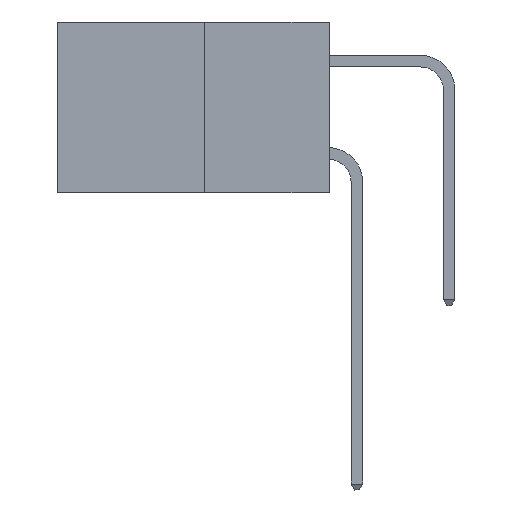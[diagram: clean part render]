
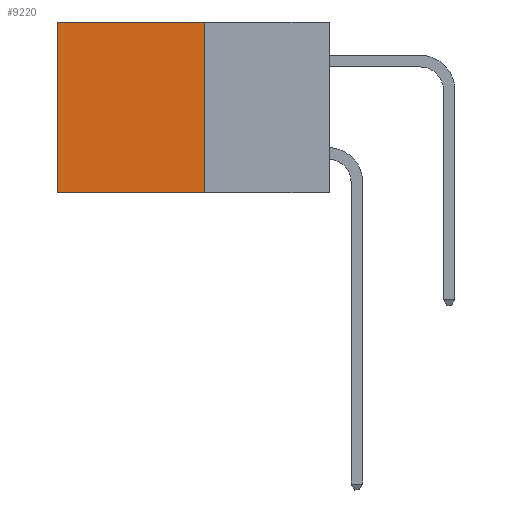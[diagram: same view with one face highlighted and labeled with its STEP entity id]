
A CAD part, left-side view. The second image highlights one B-rep face of the part: STEP entity #9220.
In plain terms, the highlighted planar face has unit normal (-1, 0, 0).
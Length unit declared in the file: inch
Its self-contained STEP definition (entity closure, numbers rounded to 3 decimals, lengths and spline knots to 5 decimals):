
#545 = VECTOR ( 'NONE', #9504, 39.37008 ) ;
#812 = LINE ( 'NONE', #10766, #545 ) ;
#907 = EDGE_CURVE ( 'NONE', #7436, #2865, #6226, .T. ) ;
#1232 = EDGE_CURVE ( 'NONE', #2865, #1827, #4604, .T. ) ;
#1278 = VECTOR ( 'NONE', #3513, 39.37008 ) ;
#1599 = CARTESIAN_POINT ( 'NONE',  ( 0.277, 0.27, 0. ) ) ;
#1723 = VERTEX_POINT ( 'NONE', #8814 ) ;
#1827 = VERTEX_POINT ( 'NONE', #4415 ) ;
#2842 = CARTESIAN_POINT ( 'NONE',  ( 0.277, 0.27, -0.37 ) ) ;
#2865 = VERTEX_POINT ( 'NONE', #7049 ) ;
#2949 = ORIENTED_EDGE ( 'NONE', *, *, #3234, .T. ) ;
#3029 = ORIENTED_EDGE ( 'NONE', *, *, #6302, .T. ) ;
#3068 = ORIENTED_EDGE ( 'NONE', *, *, #1232, .F. ) ;
#3146 = VECTOR ( 'NONE', #5377, 39.37008 ) ;
#3234 = EDGE_CURVE ( 'NONE', #7436, #1723, #812, .T. ) ;
#3513 = DIRECTION ( 'NONE',  ( 0., 0., -1. ) ) ;
#3969 = ORIENTED_EDGE ( 'NONE', *, *, #907, .F. ) ;
#4068 = FACE_OUTER_BOUND ( 'NONE', #8256, .T. ) ;
#4148 = CARTESIAN_POINT ( 'NONE',  ( 0.277, 0.27, -0.37 ) ) ;
#4415 = CARTESIAN_POINT ( 'NONE',  ( 0.277, 0.59, -0.37 ) ) ;
#4604 = LINE ( 'NONE', #2842, #8734 ) ;
#4750 = CARTESIAN_POINT ( 'NONE',  ( 0.277, 0.27, -0.37 ) ) ;
#4965 = DIRECTION ( 'NONE',  ( 1., 0., 0. ) ) ;
#5377 = DIRECTION ( 'NONE',  ( 0., 0., -1. ) ) ;
#5402 = LINE ( 'NONE', #8213, #3146 ) ;
#5996 = AXIS2_PLACEMENT_3D ( 'NONE', #4148, #4965, #10687 ) ;
#6226 = LINE ( 'NONE', #4750, #1278 ) ;
#6302 = EDGE_CURVE ( 'NONE', #1723, #1827, #5402, .T. ) ;
#7049 = CARTESIAN_POINT ( 'NONE',  ( 0.277, 0.27, -0.37 ) ) ;
#7436 = VERTEX_POINT ( 'NONE', #1599 ) ;
#7856 = DIRECTION ( 'NONE',  ( 0., 1., 0. ) ) ;
#8213 = CARTESIAN_POINT ( 'NONE',  ( 0.277, 0.59, -0.37 ) ) ;
#8256 = EDGE_LOOP ( 'NONE', ( #3029, #3068, #3969, #2949 ) ) ;
#8734 = VECTOR ( 'NONE', #7856, 39.37008 ) ;
#8814 = CARTESIAN_POINT ( 'NONE',  ( 0.277, 0.59, 0. ) ) ;
#9091 = PLANE ( 'NONE',  #5996 ) ;
#9220 = ADVANCED_FACE ( 'NONE', ( #4068 ), #9091, .F. ) ;
#9504 = DIRECTION ( 'NONE',  ( 0., 1., 0. ) ) ;
#10687 = DIRECTION ( 'NONE',  ( 0., 0., -1. ) ) ;
#10766 = CARTESIAN_POINT ( 'NONE',  ( 0.277, 0.27, 0. ) ) ;
